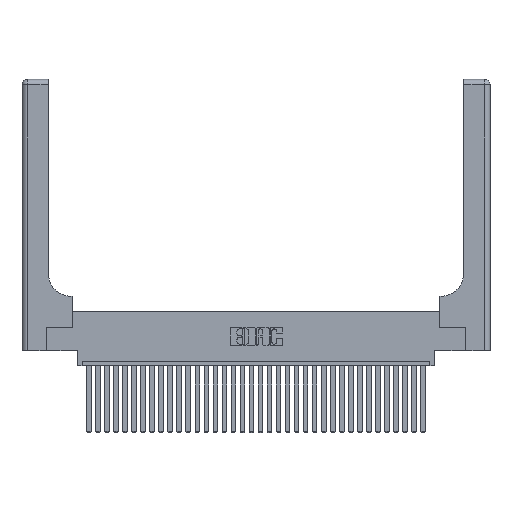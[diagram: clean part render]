
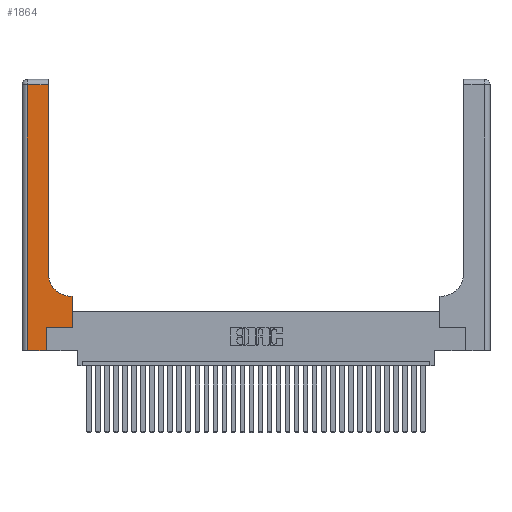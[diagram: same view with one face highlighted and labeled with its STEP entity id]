
A CAD part, top view. The second image highlights one B-rep face of the part: STEP entity #1864.
In plain terms, the highlighted planar face has unit normal (0, 0, 1).
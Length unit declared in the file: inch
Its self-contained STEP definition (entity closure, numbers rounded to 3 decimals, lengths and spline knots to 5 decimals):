
#451 = CARTESIAN_POINT ( 'NONE',  ( 0.2915, 2.94, 0.37 ) ) ;
#838 = VECTOR ( 'NONE', #13299, 39.37008 ) ;
#1571 = LINE ( 'NONE', #14400, #16041 ) ;
#1722 = VERTEX_POINT ( 'NONE', #27629 ) ;
#1864 = ADVANCED_FACE ( 'NONE', ( #30736 ), #6745, .F. ) ;
#2451 = CARTESIAN_POINT ( 'NONE',  ( 0., 2.94, 0.37 ) ) ;
#2644 = LINE ( 'NONE', #18311, #14597 ) ;
#2826 = VERTEX_POINT ( 'NONE', #28074 ) ;
#3784 = EDGE_CURVE ( 'NONE', #19033, #1722, #28974, .T. ) ;
#4174 = DIRECTION ( 'NONE',  ( 0., -1., 0. ) ) ;
#4552 = VERTEX_POINT ( 'NONE', #27380 ) ;
#4605 = AXIS2_PLACEMENT_3D ( 'NONE', #17649, #33207, #20274 ) ;
#5553 = VERTEX_POINT ( 'NONE', #17002 ) ;
#6209 = LINE ( 'NONE', #29242, #21961 ) ;
#6217 = VERTEX_POINT ( 'NONE', #10762 ) ;
#6745 = PLANE ( 'NONE',  #4605 ) ;
#8330 = VECTOR ( 'NONE', #28248, 39.37008 ) ;
#8568 = CARTESIAN_POINT ( 'NONE',  ( 0.269, 0.25, 0.37 ) ) ;
#9251 = CIRCLE ( 'NONE', #18289, 0.25 ) ;
#9259 = ORIENTED_EDGE ( 'NONE', *, *, #18044, .T. ) ;
#10559 = ORIENTED_EDGE ( 'NONE', *, *, #18139, .T. ) ;
#10762 = CARTESIAN_POINT ( 'NONE',  ( 0.5415, 0.6, 0.37 ) ) ;
#11770 = CARTESIAN_POINT ( 'NONE',  ( 0.06, 3., 0.37 ) ) ;
#13299 = DIRECTION ( 'NONE',  ( -1., 0., 0. ) ) ;
#13457 = DIRECTION ( 'NONE',  ( 1., 0., 0. ) ) ;
#14030 = DIRECTION ( 'NONE',  ( -1., 0., 0. ) ) ;
#14400 = CARTESIAN_POINT ( 'NONE',  ( 0.269, 0., 0.37 ) ) ;
#14597 = VECTOR ( 'NONE', #29121, 39.37008 ) ;
#16041 = VECTOR ( 'NONE', #16819, 39.37008 ) ;
#16249 = DIRECTION ( 'NONE',  ( 0., 0., -1. ) ) ;
#16331 = CARTESIAN_POINT ( 'NONE',  ( 0.2915, 0.6, 0.37 ) ) ;
#16819 = DIRECTION ( 'NONE',  ( 0., 1., 0. ) ) ;
#17002 = CARTESIAN_POINT ( 'NONE',  ( 0.269, 0.25, 0.37 ) ) ;
#17109 = CARTESIAN_POINT ( 'NONE',  ( 0.5585, 0.6, 0.37 ) ) ;
#17649 = CARTESIAN_POINT ( 'NONE',  ( 0., 3., 0.37 ) ) ;
#18044 = EDGE_CURVE ( 'NONE', #1722, #4552, #6209, .T. ) ;
#18093 = EDGE_CURVE ( 'NONE', #23907, #6217, #26436, .T. ) ;
#18139 = EDGE_CURVE ( 'NONE', #26348, #19033, #18658, .T. ) ;
#18289 = AXIS2_PLACEMENT_3D ( 'NONE', #21659, #16249, #21768 ) ;
#18311 = CARTESIAN_POINT ( 'NONE',  ( 0.2915, 3., 0.37 ) ) ;
#18658 = LINE ( 'NONE', #2451, #838 ) ;
#18771 = EDGE_CURVE ( 'NONE', #5553, #20427, #31405, .T. ) ;
#18997 = DIRECTION ( 'NONE',  ( 1., 0., 0. ) ) ;
#19015 = VECTOR ( 'NONE', #18997, 39.37008 ) ;
#19033 = VERTEX_POINT ( 'NONE', #25433 ) ;
#20274 = DIRECTION ( 'NONE',  ( -1., 0., 0. ) ) ;
#20427 = VERTEX_POINT ( 'NONE', #31133 ) ;
#21659 = CARTESIAN_POINT ( 'NONE',  ( 0.5415, 0.85, 0.37 ) ) ;
#21768 = DIRECTION ( 'NONE',  ( 1., 0., 0. ) ) ;
#21961 = VECTOR ( 'NONE', #13457, 39.37008 ) ;
#22004 = ORIENTED_EDGE ( 'NONE', *, *, #26373, .T. ) ;
#22877 = CARTESIAN_POINT ( 'NONE',  ( 0.5585, 0.25, 0.37 ) ) ;
#23105 = ORIENTED_EDGE ( 'NONE', *, *, #18093, .T. ) ;
#23907 = VERTEX_POINT ( 'NONE', #17109 ) ;
#24014 = ORIENTED_EDGE ( 'NONE', *, *, #26903, .T. ) ;
#24678 = ORIENTED_EDGE ( 'NONE', *, *, #18771, .T. ) ;
#24796 = VECTOR ( 'NONE', #14030, 39.37008 ) ;
#24971 = ORIENTED_EDGE ( 'NONE', *, *, #30628, .T. ) ;
#25433 = CARTESIAN_POINT ( 'NONE',  ( 0.06, 2.94, 0.37 ) ) ;
#26348 = VERTEX_POINT ( 'NONE', #451 ) ;
#26373 = EDGE_CURVE ( 'NONE', #6217, #2826, #9251, .T. ) ;
#26436 = LINE ( 'NONE', #16331, #24796 ) ;
#26476 = LINE ( 'NONE', #22877, #8330 ) ;
#26818 = ORIENTED_EDGE ( 'NONE', *, *, #3784, .T. ) ;
#26903 = EDGE_CURVE ( 'NONE', #2826, #26348, #2644, .T. ) ;
#27380 = CARTESIAN_POINT ( 'NONE',  ( 0.269, 0., 0.37 ) ) ;
#27509 = EDGE_CURVE ( 'NONE', #20427, #23907, #26476, .T. ) ;
#27629 = CARTESIAN_POINT ( 'NONE',  ( 0.06, 0., 0.37 ) ) ;
#28074 = CARTESIAN_POINT ( 'NONE',  ( 0.2915, 0.85, 0.37 ) ) ;
#28149 = VECTOR ( 'NONE', #4174, 39.37008 ) ;
#28248 = DIRECTION ( 'NONE',  ( 0., 1., 0. ) ) ;
#28974 = LINE ( 'NONE', #11770, #28149 ) ;
#29121 = DIRECTION ( 'NONE',  ( 0., 1., 0. ) ) ;
#29242 = CARTESIAN_POINT ( 'NONE',  ( 0., 0., 0.37 ) ) ;
#30628 = EDGE_CURVE ( 'NONE', #4552, #5553, #1571, .T. ) ;
#30736 = FACE_OUTER_BOUND ( 'NONE', #31224, .T. ) ;
#31133 = CARTESIAN_POINT ( 'NONE',  ( 0.5585, 0.25, 0.37 ) ) ;
#31224 = EDGE_LOOP ( 'NONE', ( #24014, #10559, #26818, #9259, #24971, #24678, #34252, #23105, #22004 ) ) ;
#31405 = LINE ( 'NONE', #8568, #19015 ) ;
#33207 = DIRECTION ( 'NONE',  ( 0., 0., -1. ) ) ;
#34252 = ORIENTED_EDGE ( 'NONE', *, *, #27509, .T. ) ;
